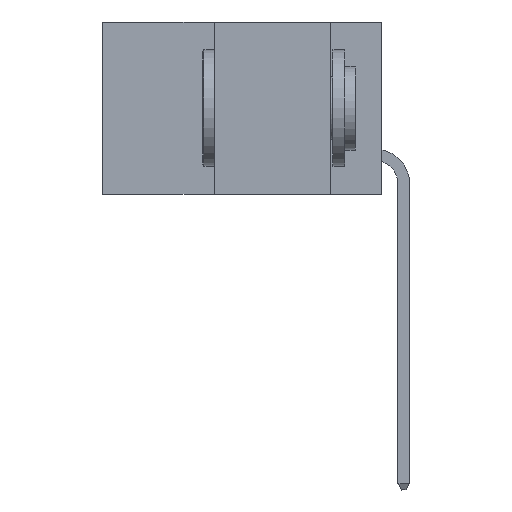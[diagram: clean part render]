
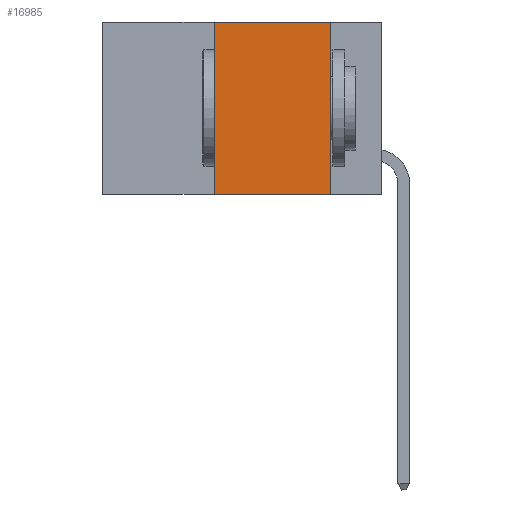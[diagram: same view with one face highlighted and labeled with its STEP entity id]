
A CAD part, left-side view. The second image highlights one B-rep face of the part: STEP entity #16985.
In plain terms, the highlighted planar face has unit normal (-1, 0, 0).
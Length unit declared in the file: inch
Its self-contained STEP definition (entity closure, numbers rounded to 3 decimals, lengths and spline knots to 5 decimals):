
#1039 = CARTESIAN_POINT ( 'NONE',  ( 0., 0.36, -0.37 ) ) ;
#1201 = DIRECTION ( 'NONE',  ( 0., 0., -1. ) ) ;
#2597 = ORIENTED_EDGE ( 'NONE', *, *, #27670, .T. ) ;
#2920 = VERTEX_POINT ( 'NONE', #1039 ) ;
#4022 = VECTOR ( 'NONE', #15030, 39.37008 ) ;
#4086 = EDGE_CURVE ( 'NONE', #8206, #18444, #26285, .T. ) ;
#4089 = CARTESIAN_POINT ( 'NONE',  ( 0., 0.6, -0.37 ) ) ;
#7170 = CARTESIAN_POINT ( 'NONE',  ( 0., 0.6, 0. ) ) ;
#7332 = LINE ( 'NONE', #27715, #17107 ) ;
#7354 = ORIENTED_EDGE ( 'NONE', *, *, #4086, .F. ) ;
#7835 = EDGE_CURVE ( 'NONE', #18444, #10634, #7332, .T. ) ;
#8206 = VERTEX_POINT ( 'NONE', #10978 ) ;
#8816 = DIRECTION ( 'NONE',  ( 0., 0., 1. ) ) ;
#9998 = DIRECTION ( 'NONE',  ( 0., 0., -1. ) ) ;
#10336 = VECTOR ( 'NONE', #21665, 39.37008 ) ;
#10634 = VERTEX_POINT ( 'NONE', #27766 ) ;
#10978 = CARTESIAN_POINT ( 'NONE',  ( 0., 0.36, 0. ) ) ;
#11072 = AXIS2_PLACEMENT_3D ( 'NONE', #7170, #18812, #1201 ) ;
#11589 = ORIENTED_EDGE ( 'NONE', *, *, #7835, .F. ) ;
#11838 = FACE_OUTER_BOUND ( 'NONE', #15642, .T. ) ;
#13998 = PLANE ( 'NONE',  #11072 ) ;
#14444 = EDGE_CURVE ( 'NONE', #2920, #8206, #22444, .T. ) ;
#15030 = DIRECTION ( 'NONE',  ( 0., -1., 0. ) ) ;
#15258 = LINE ( 'NONE', #4089, #10336 ) ;
#15642 = EDGE_LOOP ( 'NONE', ( #11589, #7354, #25403, #2597 ) ) ;
#16985 = ADVANCED_FACE ( 'NONE', ( #11838 ), #13998, .F. ) ;
#17107 = VECTOR ( 'NONE', #9998, 39.37008 ) ;
#18444 = VERTEX_POINT ( 'NONE', #24039 ) ;
#18812 = DIRECTION ( 'NONE',  ( 1., 0., 0. ) ) ;
#21665 = DIRECTION ( 'NONE',  ( 0., -1., 0. ) ) ;
#21775 = CARTESIAN_POINT ( 'NONE',  ( 0., 0.36, 0. ) ) ;
#22444 = LINE ( 'NONE', #21775, #25253 ) ;
#23948 = CARTESIAN_POINT ( 'NONE',  ( 0., 0.6, 0. ) ) ;
#24039 = CARTESIAN_POINT ( 'NONE',  ( 0., 0.11, 0. ) ) ;
#25253 = VECTOR ( 'NONE', #8816, 39.37008 ) ;
#25403 = ORIENTED_EDGE ( 'NONE', *, *, #14444, .F. ) ;
#26285 = LINE ( 'NONE', #23948, #4022 ) ;
#27670 = EDGE_CURVE ( 'NONE', #2920, #10634, #15258, .T. ) ;
#27715 = CARTESIAN_POINT ( 'NONE',  ( 0., 0.11, 0. ) ) ;
#27766 = CARTESIAN_POINT ( 'NONE',  ( 0., 0.11, -0.37 ) ) ;
